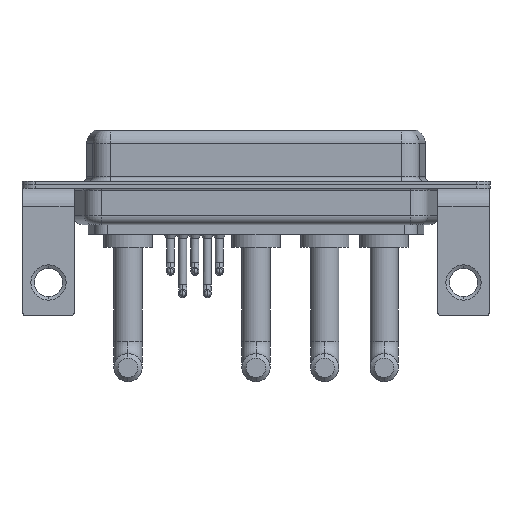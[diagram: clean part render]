
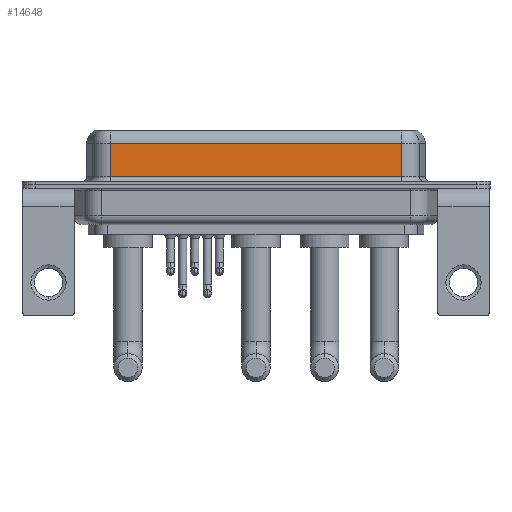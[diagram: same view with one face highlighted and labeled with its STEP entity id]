
A CAD part, front view. The second image highlights one B-rep face of the part: STEP entity #14648.
In plain terms, the highlighted planar face has unit normal (0, -1, 0).
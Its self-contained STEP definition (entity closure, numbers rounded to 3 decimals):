
#156 = CARTESIAN_POINT ( 'NONE',  ( 40.037, -3.95, 0.9 ) ) ;
#185 = VECTOR ( 'NONE', #14317, 1000. ) ;
#1158 = VECTOR ( 'NONE', #9644, 1000. ) ;
#1240 = CARTESIAN_POINT ( 'NONE',  ( 40.037, -3.95, 4.65 ) ) ;
#1340 = AXIS2_PLACEMENT_3D ( 'NONE', #10886, #16526, #15166 ) ;
#2149 = EDGE_CURVE ( 'NONE', #5430, #11246, #11866, .T. ) ;
#2596 = LINE ( 'NONE', #1240, #1158 ) ;
#2658 = FACE_OUTER_BOUND ( 'NONE', #14875, .T. ) ;
#4610 = EDGE_CURVE ( 'NONE', #5430, #12319, #2596, .T. ) ;
#5430 = VERTEX_POINT ( 'NONE', #13703 ) ;
#5638 = DIRECTION ( 'NONE',  ( 0., 0., -1. ) ) ;
#8047 = PLANE ( 'NONE',  #1340 ) ;
#8761 = CARTESIAN_POINT ( 'NONE',  ( 40.037, -3.95, 0.9 ) ) ;
#9166 = ORIENTED_EDGE ( 'NONE', *, *, #2149, .F. ) ;
#9459 = VERTEX_POINT ( 'NONE', #11540 ) ;
#9644 = DIRECTION ( 'NONE',  ( -1., 0., 0. ) ) ;
#9785 = ORIENTED_EDGE ( 'NONE', *, *, #4610, .T. ) ;
#10543 = VECTOR ( 'NONE', #5638, 1000. ) ;
#10886 = CARTESIAN_POINT ( 'NONE',  ( 40.037, -3.95, 6.4 ) ) ;
#11180 = EDGE_CURVE ( 'NONE', #12319, #9459, #12391, .T. ) ;
#11246 = VERTEX_POINT ( 'NONE', #156 ) ;
#11341 = ORIENTED_EDGE ( 'NONE', *, *, #11180, .T. ) ;
#11540 = CARTESIAN_POINT ( 'NONE',  ( 7.013, -3.95, 0.9 ) ) ;
#11866 = LINE ( 'NONE', #14957, #13923 ) ;
#12319 = VERTEX_POINT ( 'NONE', #13436 ) ;
#12391 = LINE ( 'NONE', #17948, #10543 ) ;
#13436 = CARTESIAN_POINT ( 'NONE',  ( 7.013, -3.95, 4.65 ) ) ;
#13703 = CARTESIAN_POINT ( 'NONE',  ( 40.037, -3.95, 4.65 ) ) ;
#13923 = VECTOR ( 'NONE', #17594, 1000. ) ;
#14317 = DIRECTION ( 'NONE',  ( 1., 0., 0. ) ) ;
#14648 = ADVANCED_FACE ( 'NONE', ( #2658 ), #8047, .F. ) ;
#14802 = EDGE_CURVE ( 'NONE', #9459, #11246, #15671, .T. ) ;
#14875 = EDGE_LOOP ( 'NONE', ( #9166, #9785, #11341, #15857 ) ) ;
#14957 = CARTESIAN_POINT ( 'NONE',  ( 40.037, -3.95, 6.4 ) ) ;
#15166 = DIRECTION ( 'NONE',  ( 0., 0., 1. ) ) ;
#15671 = LINE ( 'NONE', #8761, #185 ) ;
#15857 = ORIENTED_EDGE ( 'NONE', *, *, #14802, .T. ) ;
#16526 = DIRECTION ( 'NONE',  ( 0., 1., 0. ) ) ;
#17594 = DIRECTION ( 'NONE',  ( 0., 0., -1. ) ) ;
#17948 = CARTESIAN_POINT ( 'NONE',  ( 7.013, -3.95, 6.4 ) ) ;
